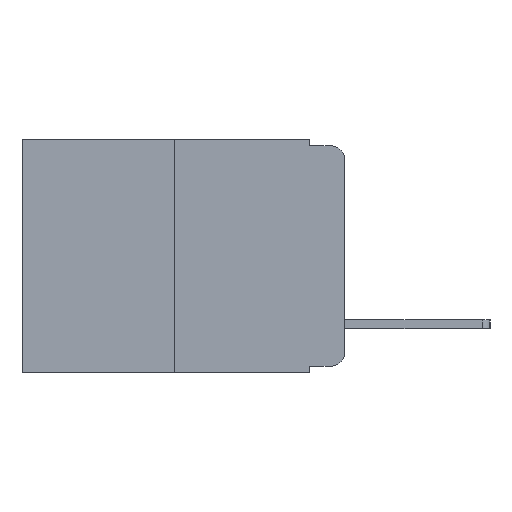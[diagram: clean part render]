
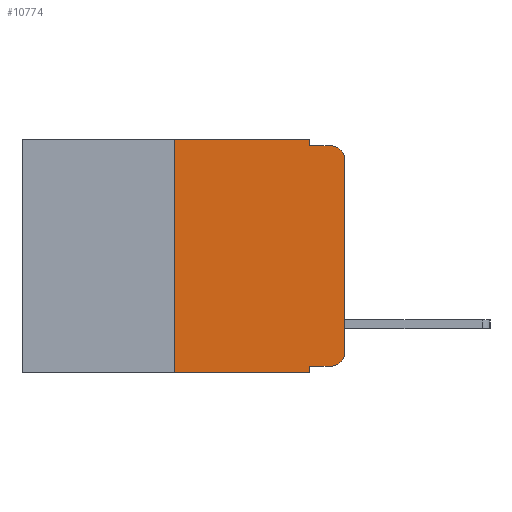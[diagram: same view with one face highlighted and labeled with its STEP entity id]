
A CAD part, left-side view. The second image highlights one B-rep face of the part: STEP entity #10774.
In plain terms, the highlighted planar face has unit normal (-1, 0, 0).
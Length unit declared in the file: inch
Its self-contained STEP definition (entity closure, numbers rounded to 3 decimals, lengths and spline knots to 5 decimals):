
#100 = PLANE ( 'NONE',  #5824 ) ;
#622 = EDGE_CURVE ( 'NONE', #6494, #7591, #1459, .T. ) ;
#819 = VECTOR ( 'NONE', #975, 39.37008 ) ;
#975 = DIRECTION ( 'NONE',  ( 0., 0., 1. ) ) ;
#991 = VERTEX_POINT ( 'NONE', #2422 ) ;
#1039 = DIRECTION ( 'NONE',  ( 0., 0., -1. ) ) ;
#1135 = LINE ( 'NONE', #10620, #10208 ) ;
#1370 = DIRECTION ( 'NONE',  ( -1., 0., 0. ) ) ;
#1373 = LINE ( 'NONE', #9954, #8706 ) ;
#1459 = LINE ( 'NONE', #10196, #8525 ) ;
#1630 = DIRECTION ( 'NONE',  ( 0., 0., 1. ) ) ;
#1792 = ORIENTED_EDGE ( 'NONE', *, *, #3751, .F. ) ;
#1946 = CARTESIAN_POINT ( 'NONE',  ( 0., 0.473, 0. ) ) ;
#1980 = EDGE_CURVE ( 'NONE', #2121, #991, #10211, .T. ) ;
#2031 = VERTEX_POINT ( 'NONE', #3162 ) ;
#2086 = CARTESIAN_POINT ( 'NONE',  ( 0., 0.25, 0. ) ) ;
#2121 = VERTEX_POINT ( 'NONE', #6750 ) ;
#2247 = VECTOR ( 'NONE', #10557, 39.37008 ) ;
#2289 = EDGE_LOOP ( 'NONE', ( #8031, #3681, #10273, #8286, #10536, #10788, #7649, #1792, #6590, #4250 ) ) ;
#2396 = CARTESIAN_POINT ( 'NONE',  ( 0., 0., 0. ) ) ;
#2422 = CARTESIAN_POINT ( 'NONE',  ( 0., 0., -0.313 ) ) ;
#2440 = CARTESIAN_POINT ( 'NONE',  ( 0., 0.051, 0. ) ) ;
#2511 = VERTEX_POINT ( 'NONE', #4889 ) ;
#2815 = DIRECTION ( 'NONE',  ( 0., -1., 0. ) ) ;
#2989 = EDGE_CURVE ( 'NONE', #6494, #6319, #5719, .T. ) ;
#3156 = VERTEX_POINT ( 'NONE', #9593 ) ;
#3162 = CARTESIAN_POINT ( 'NONE',  ( 0., 0.051, 0. ) ) ;
#3316 = VERTEX_POINT ( 'NONE', #8888 ) ;
#3350 = DIRECTION ( 'NONE',  ( 0., 0., -1. ) ) ;
#3380 = CARTESIAN_POINT ( 'NONE',  ( 0., 0.02, -0.03 ) ) ;
#3423 = CARTESIAN_POINT ( 'NONE',  ( 0., 0.051, -0.333 ) ) ;
#3681 = ORIENTED_EDGE ( 'NONE', *, *, #7823, .T. ) ;
#3751 = EDGE_CURVE ( 'NONE', #3156, #7591, #1135, .T. ) ;
#4026 = DIRECTION ( 'NONE',  ( -1., 0., 0. ) ) ;
#4250 = ORIENTED_EDGE ( 'NONE', *, *, #1980, .T. ) ;
#4524 = DIRECTION ( 'NONE',  ( 0., 0., -1. ) ) ;
#4889 = CARTESIAN_POINT ( 'NONE',  ( 0., 0.02, -0.01 ) ) ;
#5053 = CARTESIAN_POINT ( 'NONE',  ( 0., 0.473, 0. ) ) ;
#5098 = VERTEX_POINT ( 'NONE', #7957 ) ;
#5276 = DIRECTION ( 'NONE',  ( 0., 0., -1. ) ) ;
#5288 = LINE ( 'NONE', #5053, #2247 ) ;
#5664 = EDGE_CURVE ( 'NONE', #991, #5098, #5695, .T. ) ;
#5695 = LINE ( 'NONE', #2396, #9906 ) ;
#5719 = LINE ( 'NONE', #2086, #819 ) ;
#5793 = FACE_OUTER_BOUND ( 'NONE', #2289, .T. ) ;
#5824 = AXIS2_PLACEMENT_3D ( 'NONE', #1946, #6474, #1039 ) ;
#5969 = EDGE_CURVE ( 'NONE', #6319, #2031, #5288, .T. ) ;
#6062 = EDGE_CURVE ( 'NONE', #3316, #2511, #1373, .T. ) ;
#6319 = VERTEX_POINT ( 'NONE', #10357 ) ;
#6463 = AXIS2_PLACEMENT_3D ( 'NONE', #7621, #1370, #6777 ) ;
#6474 = DIRECTION ( 'NONE',  ( 1., 0., 0. ) ) ;
#6494 = VERTEX_POINT ( 'NONE', #10255 ) ;
#6590 = ORIENTED_EDGE ( 'NONE', *, *, #9376, .T. ) ;
#6620 = CARTESIAN_POINT ( 'NONE',  ( 0., 0.051, -0.343 ) ) ;
#6750 = CARTESIAN_POINT ( 'NONE',  ( 0., 0.02, -0.333 ) ) ;
#6777 = DIRECTION ( 'NONE',  ( 0., 0., -1. ) ) ;
#7136 = DIRECTION ( 'NONE',  ( 0., -1., 0. ) ) ;
#7591 = VERTEX_POINT ( 'NONE', #6620 ) ;
#7621 = CARTESIAN_POINT ( 'NONE',  ( 0., 0.02, -0.313 ) ) ;
#7642 = DIRECTION ( 'NONE',  ( 0., -1., 0. ) ) ;
#7649 = ORIENTED_EDGE ( 'NONE', *, *, #622, .T. ) ;
#7823 = EDGE_CURVE ( 'NONE', #5098, #2511, #10784, .T. ) ;
#7957 = CARTESIAN_POINT ( 'NONE',  ( 0., 0., -0.03 ) ) ;
#8031 = ORIENTED_EDGE ( 'NONE', *, *, #5664, .T. ) ;
#8112 = VECTOR ( 'NONE', #7642, 39.37008 ) ;
#8286 = ORIENTED_EDGE ( 'NONE', *, *, #11069, .F. ) ;
#8525 = VECTOR ( 'NONE', #2815, 39.37008 ) ;
#8706 = VECTOR ( 'NONE', #7136, 39.37008 ) ;
#8888 = CARTESIAN_POINT ( 'NONE',  ( 0., 0.051, -0.01 ) ) ;
#9356 = LINE ( 'NONE', #2440, #11030 ) ;
#9376 = EDGE_CURVE ( 'NONE', #3156, #2121, #10358, .T. ) ;
#9593 = CARTESIAN_POINT ( 'NONE',  ( 0., 0.051, -0.333 ) ) ;
#9906 = VECTOR ( 'NONE', #1630, 39.37008 ) ;
#9954 = CARTESIAN_POINT ( 'NONE',  ( 0., 0.051, -0.01 ) ) ;
#10196 = CARTESIAN_POINT ( 'NONE',  ( 0., 0.473, -0.343 ) ) ;
#10208 = VECTOR ( 'NONE', #5276, 39.37008 ) ;
#10211 = CIRCLE ( 'NONE', #6463, 0.02 ) ;
#10255 = CARTESIAN_POINT ( 'NONE',  ( 0., 0.25, -0.343 ) ) ;
#10273 = ORIENTED_EDGE ( 'NONE', *, *, #6062, .F. ) ;
#10357 = CARTESIAN_POINT ( 'NONE',  ( 0., 0.25, 0. ) ) ;
#10358 = LINE ( 'NONE', #3423, #8112 ) ;
#10380 = AXIS2_PLACEMENT_3D ( 'NONE', #3380, #4026, #4524 ) ;
#10536 = ORIENTED_EDGE ( 'NONE', *, *, #5969, .F. ) ;
#10557 = DIRECTION ( 'NONE',  ( 0., -1., 0. ) ) ;
#10620 = CARTESIAN_POINT ( 'NONE',  ( 0., 0.051, 0. ) ) ;
#10774 = ADVANCED_FACE ( 'NONE', ( #5793 ), #100, .F. ) ;
#10784 = CIRCLE ( 'NONE', #10380, 0.02 ) ;
#10788 = ORIENTED_EDGE ( 'NONE', *, *, #2989, .F. ) ;
#11030 = VECTOR ( 'NONE', #3350, 39.37008 ) ;
#11069 = EDGE_CURVE ( 'NONE', #2031, #3316, #9356, .T. ) ;
